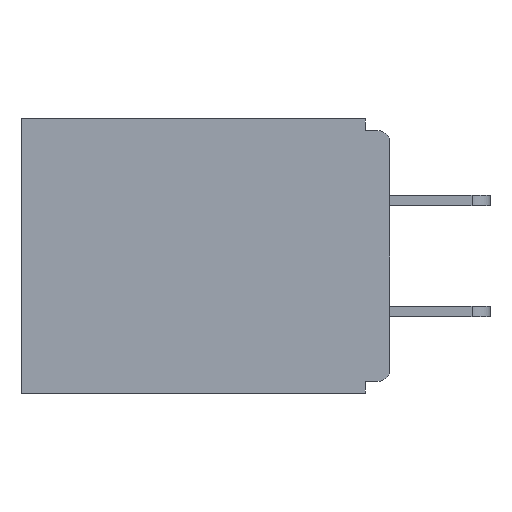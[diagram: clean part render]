
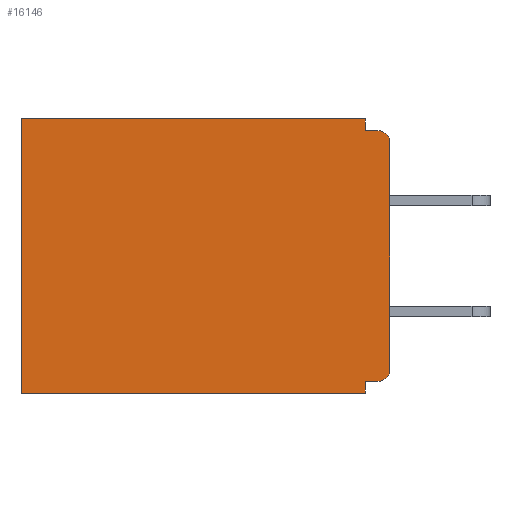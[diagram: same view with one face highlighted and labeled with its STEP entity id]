
A CAD part, left-side view. The second image highlights one B-rep face of the part: STEP entity #16146.
In plain terms, the highlighted planar face has unit normal (-1, 0, 0).
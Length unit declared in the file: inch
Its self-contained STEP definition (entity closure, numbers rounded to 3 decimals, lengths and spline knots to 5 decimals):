
#152 = DIRECTION ( 'NONE',  ( 0., 0., -1. ) ) ;
#814 = EDGE_LOOP ( 'NONE', ( #13437, #13895, #15216, #13537, #4530, #9376, #7286, #8393, #6321, #15547 ) ) ;
#1185 = DIRECTION ( 'NONE',  ( 0., -1., 0. ) ) ;
#1253 = DIRECTION ( 'NONE',  ( 0., 0., -1. ) ) ;
#1692 = EDGE_CURVE ( 'NONE', #9302, #15505, #14266, .T. ) ;
#2196 = LINE ( 'NONE', #4954, #12364 ) ;
#2367 = CARTESIAN_POINT ( 'NONE',  ( 0.298, 0.015, -0.03 ) ) ;
#2712 = VERTEX_POINT ( 'NONE', #14222 ) ;
#3063 = LINE ( 'NONE', #14554, #18307 ) ;
#3529 = CARTESIAN_POINT ( 'NONE',  ( 0.298, 0.015, -0.313 ) ) ;
#3577 = EDGE_CURVE ( 'NONE', #18253, #17810, #13745, .T. ) ;
#3781 = EDGE_CURVE ( 'NONE', #18253, #6369, #4973, .T. ) ;
#4035 = VECTOR ( 'NONE', #13989, 39.37008 ) ;
#4210 = AXIS2_PLACEMENT_3D ( 'NONE', #2367, #14003, #12694 ) ;
#4530 = ORIENTED_EDGE ( 'NONE', *, *, #16392, .T. ) ;
#4665 = VECTOR ( 'NONE', #5852, 39.37008 ) ;
#4954 = CARTESIAN_POINT ( 'NONE',  ( 0.298, 0., 0. ) ) ;
#4973 = LINE ( 'NONE', #8183, #4035 ) ;
#4989 = EDGE_CURVE ( 'NONE', #10269, #16041, #7219, .T. ) ;
#5046 = CARTESIAN_POINT ( 'NONE',  ( 0.298, 0., 0. ) ) ;
#5070 = VERTEX_POINT ( 'NONE', #17842 ) ;
#5498 = EDGE_CURVE ( 'NONE', #10375, #2712, #18709, .T. ) ;
#5852 = DIRECTION ( 'NONE',  ( 0., 1., 0. ) ) ;
#5903 = CARTESIAN_POINT ( 'NONE',  ( 0.298, 0.031, 0. ) ) ;
#6190 = CARTESIAN_POINT ( 'NONE',  ( 0.298, 0., -0.03 ) ) ;
#6213 = CARTESIAN_POINT ( 'NONE',  ( 0.298, 0., -0.343 ) ) ;
#6321 = ORIENTED_EDGE ( 'NONE', *, *, #3577, .T. ) ;
#6369 = VERTEX_POINT ( 'NONE', #18295 ) ;
#6447 = DIRECTION ( 'NONE',  ( -1., 0., 0. ) ) ;
#6474 = FACE_OUTER_BOUND ( 'NONE', #814, .T. ) ;
#7211 = CARTESIAN_POINT ( 'NONE',  ( 0.298, 0., -0.015 ) ) ;
#7219 = LINE ( 'NONE', #6213, #4665 ) ;
#7286 = ORIENTED_EDGE ( 'NONE', *, *, #8863, .F. ) ;
#7986 = VECTOR ( 'NONE', #8520, 39.37008 ) ;
#8183 = CARTESIAN_POINT ( 'NONE',  ( 0.298, 0., -0.328 ) ) ;
#8393 = ORIENTED_EDGE ( 'NONE', *, *, #3781, .F. ) ;
#8520 = DIRECTION ( 'NONE',  ( 0., 0., -1. ) ) ;
#8671 = LINE ( 'NONE', #18812, #7986 ) ;
#8863 = EDGE_CURVE ( 'NONE', #6369, #10269, #8671, .T. ) ;
#8951 = EDGE_CURVE ( 'NONE', #9302, #17810, #2196, .T. ) ;
#9254 = VECTOR ( 'NONE', #152, 39.37008 ) ;
#9302 = VERTEX_POINT ( 'NONE', #6190 ) ;
#9330 = CARTESIAN_POINT ( 'NONE',  ( 0.298, 0., -0.313 ) ) ;
#9376 = ORIENTED_EDGE ( 'NONE', *, *, #4989, .F. ) ;
#9999 = DIRECTION ( 'NONE',  ( 0., 1., 0. ) ) ;
#10167 = AXIS2_PLACEMENT_3D ( 'NONE', #5046, #15380, #16846 ) ;
#10269 = VERTEX_POINT ( 'NONE', #14234 ) ;
#10375 = VERTEX_POINT ( 'NONE', #5903 ) ;
#12245 = DIRECTION ( 'NONE',  ( 0., 0., -1. ) ) ;
#12364 = VECTOR ( 'NONE', #13002, 39.37008 ) ;
#12694 = DIRECTION ( 'NONE',  ( 0., 0., -1. ) ) ;
#13002 = DIRECTION ( 'NONE',  ( 0., 0., -1. ) ) ;
#13437 = ORIENTED_EDGE ( 'NONE', *, *, #1692, .T. ) ;
#13532 = CARTESIAN_POINT ( 'NONE',  ( 0.298, 0.46, 0. ) ) ;
#13537 = ORIENTED_EDGE ( 'NONE', *, *, #5498, .T. ) ;
#13681 = CARTESIAN_POINT ( 'NONE',  ( 0.298, 0., 0. ) ) ;
#13745 = CIRCLE ( 'NONE', #15498, 0.015 ) ;
#13834 = EDGE_CURVE ( 'NONE', #5070, #15505, #15063, .T. ) ;
#13850 = LINE ( 'NONE', #13532, #9254 ) ;
#13877 = PLANE ( 'NONE',  #10167 ) ;
#13895 = ORIENTED_EDGE ( 'NONE', *, *, #13834, .F. ) ;
#13954 = EDGE_CURVE ( 'NONE', #10375, #5070, #3063, .T. ) ;
#13989 = DIRECTION ( 'NONE',  ( 0., 1., 0. ) ) ;
#14003 = DIRECTION ( 'NONE',  ( -1., 0., 0. ) ) ;
#14222 = CARTESIAN_POINT ( 'NONE',  ( 0.298, 0.46, 0. ) ) ;
#14234 = CARTESIAN_POINT ( 'NONE',  ( 0.298, 0.031, -0.343 ) ) ;
#14266 = CIRCLE ( 'NONE', #4210, 0.015 ) ;
#14554 = CARTESIAN_POINT ( 'NONE',  ( 0.298, 0.031, -0.343 ) ) ;
#14721 = CARTESIAN_POINT ( 'NONE',  ( 0.298, 0.015, -0.328 ) ) ;
#15063 = LINE ( 'NONE', #7211, #17845 ) ;
#15216 = ORIENTED_EDGE ( 'NONE', *, *, #13954, .F. ) ;
#15380 = DIRECTION ( 'NONE',  ( 1., 0., 0. ) ) ;
#15414 = CARTESIAN_POINT ( 'NONE',  ( 0.298, 0.015, -0.015 ) ) ;
#15498 = AXIS2_PLACEMENT_3D ( 'NONE', #3529, #6447, #12245 ) ;
#15505 = VERTEX_POINT ( 'NONE', #15414 ) ;
#15547 = ORIENTED_EDGE ( 'NONE', *, *, #8951, .F. ) ;
#16041 = VERTEX_POINT ( 'NONE', #17249 ) ;
#16146 = ADVANCED_FACE ( 'NONE', ( #6474 ), #13877, .F. ) ;
#16392 = EDGE_CURVE ( 'NONE', #2712, #16041, #13850, .T. ) ;
#16846 = DIRECTION ( 'NONE',  ( 0., 0., -1. ) ) ;
#17249 = CARTESIAN_POINT ( 'NONE',  ( 0.298, 0.46, -0.343 ) ) ;
#17810 = VERTEX_POINT ( 'NONE', #9330 ) ;
#17842 = CARTESIAN_POINT ( 'NONE',  ( 0.298, 0.031, -0.015 ) ) ;
#17845 = VECTOR ( 'NONE', #1185, 39.37008 ) ;
#18253 = VERTEX_POINT ( 'NONE', #14721 ) ;
#18295 = CARTESIAN_POINT ( 'NONE',  ( 0.298, 0.031, -0.328 ) ) ;
#18307 = VECTOR ( 'NONE', #1253, 39.37008 ) ;
#18501 = VECTOR ( 'NONE', #9999, 39.37008 ) ;
#18709 = LINE ( 'NONE', #13681, #18501 ) ;
#18812 = CARTESIAN_POINT ( 'NONE',  ( 0.298, 0.031, -0.343 ) ) ;
